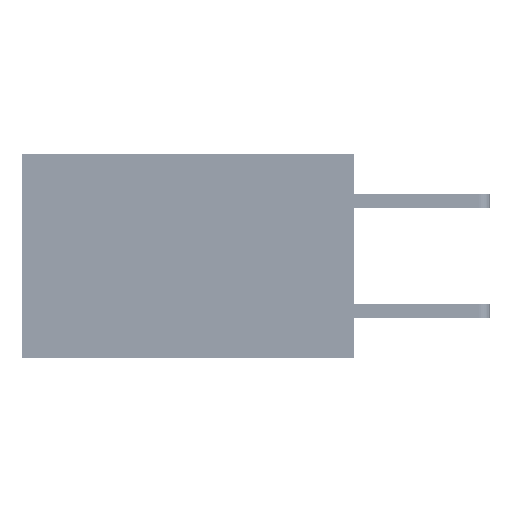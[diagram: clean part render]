
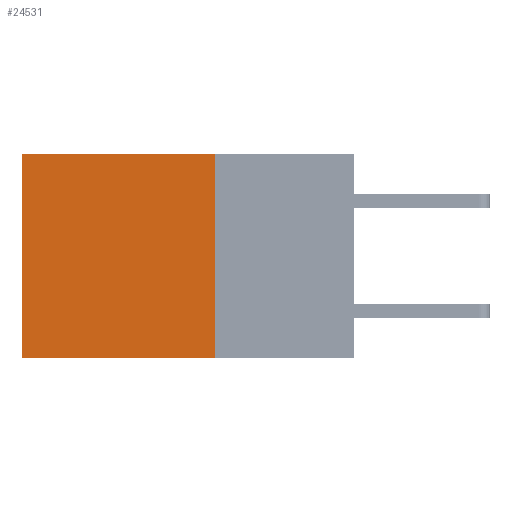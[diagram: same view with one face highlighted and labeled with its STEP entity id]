
A CAD part, left-side view. The second image highlights one B-rep face of the part: STEP entity #24531.
In plain terms, the highlighted planar face has unit normal (-1, 0, 0).
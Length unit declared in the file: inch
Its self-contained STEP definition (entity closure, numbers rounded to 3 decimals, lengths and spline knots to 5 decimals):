
#831 = DIRECTION ( 'NONE',  ( 1., 0., 0. ) ) ;
#3672 = VECTOR ( 'NONE', #27966, 39.37008 ) ;
#4191 = EDGE_CURVE ( 'NONE', #28868, #23899, #27954, .T. ) ;
#4627 = VECTOR ( 'NONE', #10758, 39.37008 ) ;
#5514 = DIRECTION ( 'NONE',  ( 0., 0., -1. ) ) ;
#6096 = ORIENTED_EDGE ( 'NONE', *, *, #37242, .F. ) ;
#6106 = DIRECTION ( 'NONE',  ( 0., 1., 0. ) ) ;
#6422 = ORIENTED_EDGE ( 'NONE', *, *, #9437, .T. ) ;
#6726 = AXIS2_PLACEMENT_3D ( 'NONE', #42880, #831, #28789 ) ;
#6974 = VERTEX_POINT ( 'NONE', #8416 ) ;
#8087 = CARTESIAN_POINT ( 'NONE',  ( 0.2875, 0.6, 0. ) ) ;
#8416 = CARTESIAN_POINT ( 'NONE',  ( 0.2875, 0.25, -0.37 ) ) ;
#9437 = EDGE_CURVE ( 'NONE', #23899, #42623, #26376, .T. ) ;
#10758 = DIRECTION ( 'NONE',  ( 0., 1., 0. ) ) ;
#11273 = VECTOR ( 'NONE', #5514, 39.37008 ) ;
#14795 = ORIENTED_EDGE ( 'NONE', *, *, #4191, .T. ) ;
#15770 = EDGE_CURVE ( 'NONE', #6974, #42623, #35109, .T. ) ;
#18096 = PLANE ( 'NONE',  #6726 ) ;
#18349 = FACE_OUTER_BOUND ( 'NONE', #39151, .T. ) ;
#21943 = VECTOR ( 'NONE', #6106, 39.37008 ) ;
#22899 = CARTESIAN_POINT ( 'NONE',  ( 0.2875, 0.25, 0. ) ) ;
#23899 = VERTEX_POINT ( 'NONE', #8087 ) ;
#24396 = CARTESIAN_POINT ( 'NONE',  ( 0.2875, 0.6, 0. ) ) ;
#24531 = ADVANCED_FACE ( 'NONE', ( #18349 ), #18096, .F. ) ;
#26376 = LINE ( 'NONE', #24396, #3672 ) ;
#27954 = LINE ( 'NONE', #22899, #21943 ) ;
#27966 = DIRECTION ( 'NONE',  ( 0., 0., -1. ) ) ;
#28558 = CARTESIAN_POINT ( 'NONE',  ( 0.2875, 0.25, -0.37 ) ) ;
#28789 = DIRECTION ( 'NONE',  ( 0., 0., -1. ) ) ;
#28868 = VERTEX_POINT ( 'NONE', #37536 ) ;
#33414 = CARTESIAN_POINT ( 'NONE',  ( 0.2875, 0.25, 0. ) ) ;
#35109 = LINE ( 'NONE', #28558, #4627 ) ;
#35641 = LINE ( 'NONE', #33414, #11273 ) ;
#37242 = EDGE_CURVE ( 'NONE', #28868, #6974, #35641, .T. ) ;
#37536 = CARTESIAN_POINT ( 'NONE',  ( 0.2875, 0.25, 0. ) ) ;
#39151 = EDGE_LOOP ( 'NONE', ( #6422, #45204, #6096, #14795 ) ) ;
#41981 = CARTESIAN_POINT ( 'NONE',  ( 0.2875, 0.6, -0.37 ) ) ;
#42623 = VERTEX_POINT ( 'NONE', #41981 ) ;
#42880 = CARTESIAN_POINT ( 'NONE',  ( 0.2875, 0.25, 0. ) ) ;
#45204 = ORIENTED_EDGE ( 'NONE', *, *, #15770, .F. ) ;
